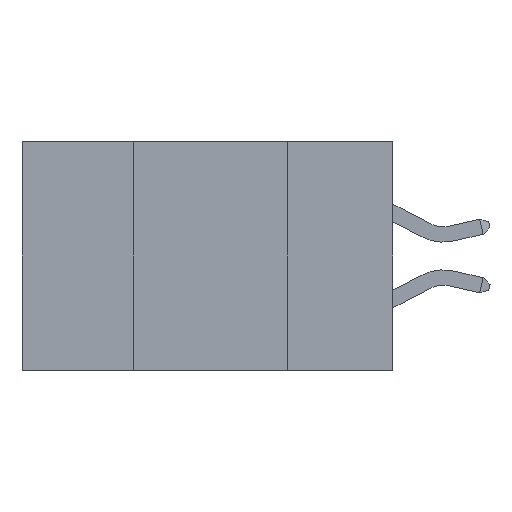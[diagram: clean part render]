
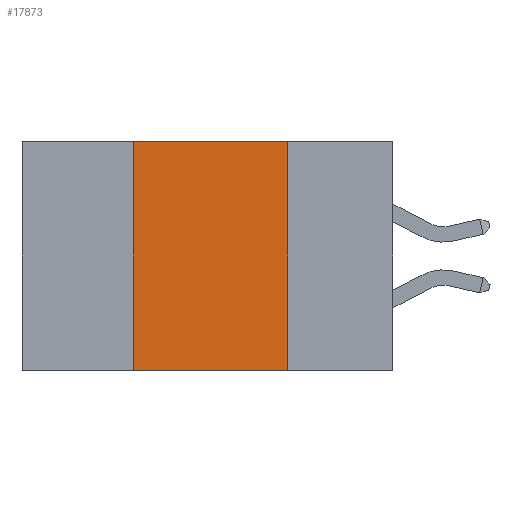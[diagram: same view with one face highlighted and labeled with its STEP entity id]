
A CAD part, left-side view. The second image highlights one B-rep face of the part: STEP entity #17873.
In plain terms, the highlighted planar face has unit normal (-1, 0, 0).
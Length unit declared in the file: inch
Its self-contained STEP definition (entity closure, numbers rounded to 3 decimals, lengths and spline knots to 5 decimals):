
#1232 = EDGE_CURVE ( 'NONE', #14458, #6018, #5390, .T. ) ;
#1262 = FACE_OUTER_BOUND ( 'NONE', #25400, .T. ) ;
#3286 = VECTOR ( 'NONE', #18161, 39.37008 ) ;
#3550 = LINE ( 'NONE', #19152, #24156 ) ;
#3932 = LINE ( 'NONE', #24177, #3286 ) ;
#4244 = PLANE ( 'NONE',  #7006 ) ;
#4769 = CARTESIAN_POINT ( 'NONE',  ( 0., 0.6, -0.37 ) ) ;
#4927 = CARTESIAN_POINT ( 'NONE',  ( 0., 0.17, 0. ) ) ;
#5355 = EDGE_CURVE ( 'NONE', #7128, #6847, #14353, .T. ) ;
#5390 = LINE ( 'NONE', #24224, #18607 ) ;
#5917 = ORIENTED_EDGE ( 'NONE', *, *, #23681, .F. ) ;
#6018 = VERTEX_POINT ( 'NONE', #4927 ) ;
#6690 = ORIENTED_EDGE ( 'NONE', *, *, #5355, .T. ) ;
#6847 = VERTEX_POINT ( 'NONE', #24739 ) ;
#7006 = AXIS2_PLACEMENT_3D ( 'NONE', #24437, #14189, #16257 ) ;
#7128 = VERTEX_POINT ( 'NONE', #22044 ) ;
#12729 = VECTOR ( 'NONE', #12796, 39.37008 ) ;
#12796 = DIRECTION ( 'NONE',  ( 0., -1., 0. ) ) ;
#13396 = EDGE_CURVE ( 'NONE', #6018, #6847, #3932, .T. ) ;
#14189 = DIRECTION ( 'NONE',  ( 1., 0., 0. ) ) ;
#14353 = LINE ( 'NONE', #4769, #12729 ) ;
#14458 = VERTEX_POINT ( 'NONE', #15465 ) ;
#15465 = CARTESIAN_POINT ( 'NONE',  ( 0., 0.42, 0. ) ) ;
#16054 = DIRECTION ( 'NONE',  ( 0., -1., 0. ) ) ;
#16257 = DIRECTION ( 'NONE',  ( 0., 0., -1. ) ) ;
#17546 = ORIENTED_EDGE ( 'NONE', *, *, #1232, .F. ) ;
#17873 = ADVANCED_FACE ( 'NONE', ( #1262 ), #4244, .F. ) ;
#18161 = DIRECTION ( 'NONE',  ( 0., 0., -1. ) ) ;
#18607 = VECTOR ( 'NONE', #16054, 39.37008 ) ;
#19152 = CARTESIAN_POINT ( 'NONE',  ( 0., 0.42, 0. ) ) ;
#22044 = CARTESIAN_POINT ( 'NONE',  ( 0., 0.42, -0.37 ) ) ;
#22642 = ORIENTED_EDGE ( 'NONE', *, *, #13396, .F. ) ;
#23681 = EDGE_CURVE ( 'NONE', #7128, #14458, #3550, .T. ) ;
#23689 = DIRECTION ( 'NONE',  ( 0., 0., 1. ) ) ;
#24156 = VECTOR ( 'NONE', #23689, 39.37008 ) ;
#24177 = CARTESIAN_POINT ( 'NONE',  ( 0., 0.17, 0. ) ) ;
#24224 = CARTESIAN_POINT ( 'NONE',  ( 0., 0.6, 0. ) ) ;
#24437 = CARTESIAN_POINT ( 'NONE',  ( 0., 0.6, 0. ) ) ;
#24739 = CARTESIAN_POINT ( 'NONE',  ( 0., 0.17, -0.37 ) ) ;
#25400 = EDGE_LOOP ( 'NONE', ( #22642, #17546, #5917, #6690 ) ) ;
